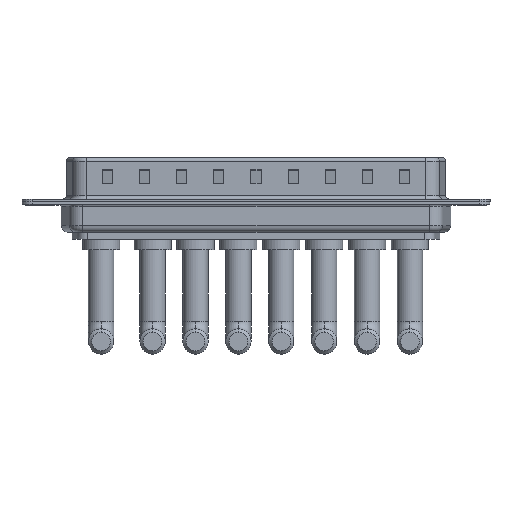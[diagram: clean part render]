
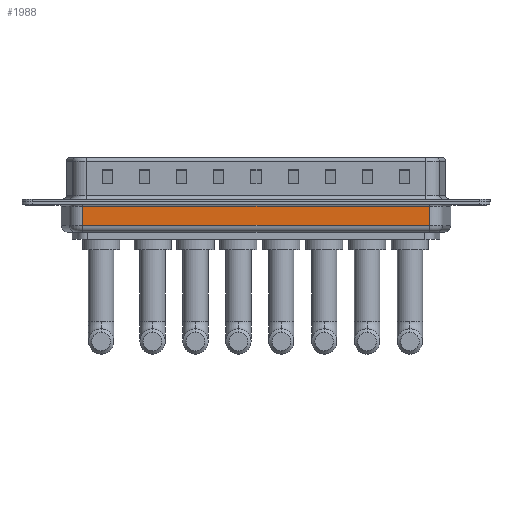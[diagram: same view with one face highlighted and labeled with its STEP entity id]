
A CAD part, front view. The second image highlights one B-rep face of the part: STEP entity #1988.
In plain terms, the highlighted planar face has unit normal (0, -1, 0).
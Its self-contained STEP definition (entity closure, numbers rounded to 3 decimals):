
#179 = VERTEX_POINT ( 'NONE', #9866 ) ;
#485 = VERTEX_POINT ( 'NONE', #8346 ) ;
#634 = EDGE_LOOP ( 'NONE', ( #12893, #4685, #805, #954 ) ) ;
#805 = ORIENTED_EDGE ( 'NONE', *, *, #11212, .T. ) ;
#954 = ORIENTED_EDGE ( 'NONE', *, *, #1708, .T. ) ;
#1309 = DIRECTION ( 'NONE',  ( -1., 0., 0. ) ) ;
#1467 = LINE ( 'NONE', #13695, #7804 ) ;
#1708 = EDGE_CURVE ( 'NONE', #13400, #9435, #3054, .T. ) ;
#1988 = ADVANCED_FACE ( 'NONE', ( #11223 ), #3478, .F. ) ;
#2493 = VECTOR ( 'NONE', #5306, 1000. ) ;
#2830 = CARTESIAN_POINT ( 'NONE',  ( 6.031, -5.35, -0.65 ) ) ;
#3054 = LINE ( 'NONE', #2830, #10919 ) ;
#3478 = PLANE ( 'NONE',  #7691 ) ;
#4685 = ORIENTED_EDGE ( 'NONE', *, *, #8191, .T. ) ;
#4752 = CARTESIAN_POINT ( 'NONE',  ( 57.469, -5.35, -0.65 ) ) ;
#5306 = DIRECTION ( 'NONE',  ( 0., 0., 1. ) ) ;
#5798 = LINE ( 'NONE', #11029, #6670 ) ;
#6317 = CARTESIAN_POINT ( 'NONE',  ( 6.031, -5.35, -4.5 ) ) ;
#6670 = VECTOR ( 'NONE', #9145, 1000. ) ;
#7389 = EDGE_CURVE ( 'NONE', #485, #9435, #8792, .T. ) ;
#7691 = AXIS2_PLACEMENT_3D ( 'NONE', #8034, #9272, #1309 ) ;
#7804 = VECTOR ( 'NONE', #13556, 1000. ) ;
#8034 = CARTESIAN_POINT ( 'NONE',  ( 6.031, -5.35, -4.5 ) ) ;
#8191 = EDGE_CURVE ( 'NONE', #485, #179, #1467, .T. ) ;
#8346 = CARTESIAN_POINT ( 'NONE',  ( 6.031, -5.35, -3.5 ) ) ;
#8792 = LINE ( 'NONE', #6317, #2493 ) ;
#8884 = CARTESIAN_POINT ( 'NONE',  ( 6.031, -5.35, -0.65 ) ) ;
#9145 = DIRECTION ( 'NONE',  ( 0., 0., 1. ) ) ;
#9272 = DIRECTION ( 'NONE',  ( 0., 1., 0. ) ) ;
#9435 = VERTEX_POINT ( 'NONE', #8884 ) ;
#9866 = CARTESIAN_POINT ( 'NONE',  ( 57.469, -5.35, -3.5 ) ) ;
#10919 = VECTOR ( 'NONE', #12987, 1000. ) ;
#11029 = CARTESIAN_POINT ( 'NONE',  ( 57.469, -5.35, -4.5 ) ) ;
#11212 = EDGE_CURVE ( 'NONE', #179, #13400, #5798, .T. ) ;
#11223 = FACE_OUTER_BOUND ( 'NONE', #634, .T. ) ;
#12893 = ORIENTED_EDGE ( 'NONE', *, *, #7389, .F. ) ;
#12987 = DIRECTION ( 'NONE',  ( -1., 0., 0. ) ) ;
#13400 = VERTEX_POINT ( 'NONE', #4752 ) ;
#13556 = DIRECTION ( 'NONE',  ( 1., 0., 0. ) ) ;
#13695 = CARTESIAN_POINT ( 'NONE',  ( 6.031, -5.35, -3.5 ) ) ;
